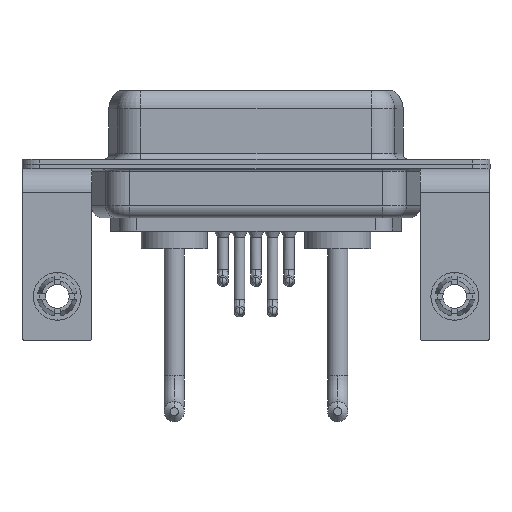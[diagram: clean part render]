
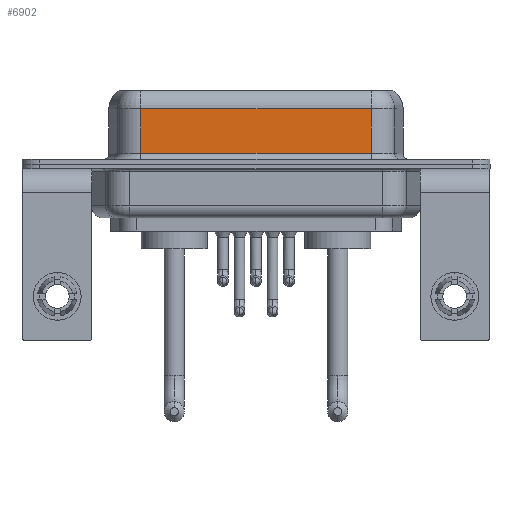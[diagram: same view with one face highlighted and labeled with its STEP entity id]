
A CAD part, front view. The second image highlights one B-rep face of the part: STEP entity #6902.
In plain terms, the highlighted planar face has unit normal (0, -1, 0).
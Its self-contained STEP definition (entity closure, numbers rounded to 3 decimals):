
#273 = VECTOR ( 'NONE', #7607, 1000. ) ;
#1005 = AXIS2_PLACEMENT_3D ( 'NONE', #4124, #12722, #2666 ) ;
#1106 = FACE_OUTER_BOUND ( 'NONE', #8312, .T. ) ;
#1801 = EDGE_CURVE ( 'NONE', #5688, #14741, #13554, .T. ) ;
#2666 = DIRECTION ( 'NONE',  ( 0., 0., 1. ) ) ;
#3636 = CARTESIAN_POINT ( 'NONE',  ( 7.013, -3.95, 6.4 ) ) ;
#4124 = CARTESIAN_POINT ( 'NONE',  ( 26.287, -3.95, 6.4 ) ) ;
#4291 = VECTOR ( 'NONE', #9402, 1000. ) ;
#5688 = VERTEX_POINT ( 'NONE', #10667 ) ;
#6090 = LINE ( 'NONE', #10866, #4291 ) ;
#6289 = VERTEX_POINT ( 'NONE', #14322 ) ;
#6779 = PLANE ( 'NONE',  #1005 ) ;
#6888 = ORIENTED_EDGE ( 'NONE', *, *, #13520, .T. ) ;
#6902 = ADVANCED_FACE ( 'NONE', ( #1106 ), #6779, .F. ) ;
#7607 = DIRECTION ( 'NONE',  ( -1., 0., 0. ) ) ;
#8312 = EDGE_LOOP ( 'NONE', ( #15443, #17232, #6888, #18564 ) ) ;
#8462 = CARTESIAN_POINT ( 'NONE',  ( 26.287, -3.95, 6.4 ) ) ;
#9125 = VECTOR ( 'NONE', #11161, 1000. ) ;
#9402 = DIRECTION ( 'NONE',  ( 1., 0., 0. ) ) ;
#10667 = CARTESIAN_POINT ( 'NONE',  ( 26.287, -3.95, 4.65 ) ) ;
#10835 = CARTESIAN_POINT ( 'NONE',  ( 26.287, -3.95, 4.65 ) ) ;
#10866 = CARTESIAN_POINT ( 'NONE',  ( 26.287, -3.95, 0.9 ) ) ;
#11161 = DIRECTION ( 'NONE',  ( 0., 0., -1. ) ) ;
#11489 = DIRECTION ( 'NONE',  ( 0., 0., -1. ) ) ;
#12722 = DIRECTION ( 'NONE',  ( 0., 1., 0. ) ) ;
#12775 = EDGE_CURVE ( 'NONE', #5688, #6289, #14783, .T. ) ;
#13341 = VECTOR ( 'NONE', #11489, 1000. ) ;
#13520 = EDGE_CURVE ( 'NONE', #14741, #16048, #13965, .T. ) ;
#13554 = LINE ( 'NONE', #10835, #273 ) ;
#13965 = LINE ( 'NONE', #3636, #9125 ) ;
#14322 = CARTESIAN_POINT ( 'NONE',  ( 26.287, -3.95, 0.9 ) ) ;
#14741 = VERTEX_POINT ( 'NONE', #15517 ) ;
#14783 = LINE ( 'NONE', #8462, #13341 ) ;
#15443 = ORIENTED_EDGE ( 'NONE', *, *, #12775, .F. ) ;
#15517 = CARTESIAN_POINT ( 'NONE',  ( 7.013, -3.95, 4.65 ) ) ;
#16048 = VERTEX_POINT ( 'NONE', #18963 ) ;
#17232 = ORIENTED_EDGE ( 'NONE', *, *, #1801, .T. ) ;
#18564 = ORIENTED_EDGE ( 'NONE', *, *, #18980, .T. ) ;
#18963 = CARTESIAN_POINT ( 'NONE',  ( 7.013, -3.95, 0.9 ) ) ;
#18980 = EDGE_CURVE ( 'NONE', #16048, #6289, #6090, .T. ) ;
